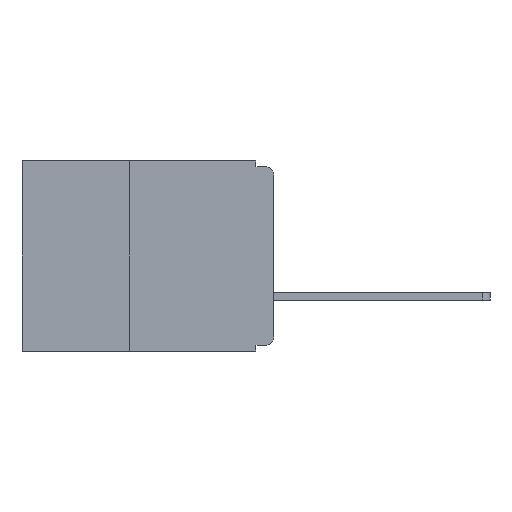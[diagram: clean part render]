
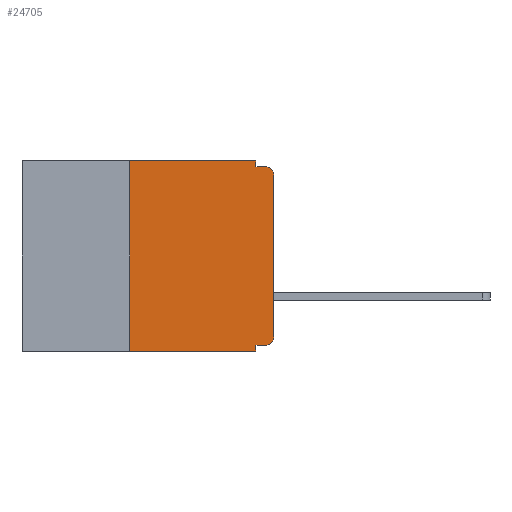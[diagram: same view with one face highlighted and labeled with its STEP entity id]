
A CAD part, left-side view. The second image highlights one B-rep face of the part: STEP entity #24705.
In plain terms, the highlighted planar face has unit normal (-1, 0, 0).
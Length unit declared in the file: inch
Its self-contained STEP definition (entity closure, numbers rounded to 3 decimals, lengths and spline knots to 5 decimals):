
#12 = CARTESIAN_POINT ( 'NONE',  ( 0., 0.031, -0.01 ) ) ;
#156 = VERTEX_POINT ( 'NONE', #18353 ) ;
#365 = EDGE_CURVE ( 'NONE', #24857, #156, #10407, .T. ) ;
#475 = ORIENTED_EDGE ( 'NONE', *, *, #11250, .T. ) ;
#1163 = VERTEX_POINT ( 'NONE', #9125 ) ;
#1238 = AXIS2_PLACEMENT_3D ( 'NONE', #21789, #4111, #19715 ) ;
#1511 = CARTESIAN_POINT ( 'NONE',  ( 0., 0., -0.01 ) ) ;
#2119 = DIRECTION ( 'NONE',  ( 0., 0., 1. ) ) ;
#2271 = FACE_OUTER_BOUND ( 'NONE', #23201, .T. ) ;
#2427 = EDGE_CURVE ( 'NONE', #20034, #23297, #3853, .T. ) ;
#2772 = CIRCLE ( 'NONE', #10408, 0.015 ) ;
#2891 = VERTEX_POINT ( 'NONE', #18834 ) ;
#3417 = CARTESIAN_POINT ( 'NONE',  ( 0., 0.437, 0. ) ) ;
#3722 = ORIENTED_EDGE ( 'NONE', *, *, #5728, .T. ) ;
#3853 = LINE ( 'NONE', #24608, #10629 ) ;
#4111 = DIRECTION ( 'NONE',  ( 1., 0., 0. ) ) ;
#4573 = LINE ( 'NONE', #6805, #6740 ) ;
#4807 = CARTESIAN_POINT ( 'NONE',  ( 0., 0.015, -0.305 ) ) ;
#5728 = EDGE_CURVE ( 'NONE', #15948, #16632, #4573, .T. ) ;
#5747 = VECTOR ( 'NONE', #25563, 39.37008 ) ;
#6016 = ORIENTED_EDGE ( 'NONE', *, *, #365, .F. ) ;
#6680 = CARTESIAN_POINT ( 'NONE',  ( 0., 0.25, -0.33 ) ) ;
#6740 = VECTOR ( 'NONE', #2119, 39.37008 ) ;
#6805 = CARTESIAN_POINT ( 'NONE',  ( 0., 0., 0. ) ) ;
#7125 = CARTESIAN_POINT ( 'NONE',  ( 0., 0., -0.025 ) ) ;
#7126 = DIRECTION ( 'NONE',  ( 0., 0., -1. ) ) ;
#7521 = DIRECTION ( 'NONE',  ( -1., 0., 0. ) ) ;
#8310 = LINE ( 'NONE', #8464, #13542 ) ;
#8464 = CARTESIAN_POINT ( 'NONE',  ( 0., 0.437, -0.33 ) ) ;
#9125 = CARTESIAN_POINT ( 'NONE',  ( 0., 0.031, -0.33 ) ) ;
#9532 = EDGE_CURVE ( 'NONE', #2891, #18909, #24027, .T. ) ;
#10407 = LINE ( 'NONE', #26718, #21393 ) ;
#10408 = AXIS2_PLACEMENT_3D ( 'NONE', #4807, #20368, #7126 ) ;
#10629 = VECTOR ( 'NONE', #24596, 39.37008 ) ;
#11250 = EDGE_CURVE ( 'NONE', #24857, #15948, #2772, .T. ) ;
#11747 = LINE ( 'NONE', #3417, #5747 ) ;
#12354 = ORIENTED_EDGE ( 'NONE', *, *, #22501, .F. ) ;
#12846 = LINE ( 'NONE', #1511, #18021 ) ;
#12863 = DIRECTION ( 'NONE',  ( 0., -1., 0. ) ) ;
#12937 = DIRECTION ( 'NONE',  ( 0., -1., 0. ) ) ;
#13099 = PLANE ( 'NONE',  #1238 ) ;
#13159 = CARTESIAN_POINT ( 'NONE',  ( 0., 0.25, 0. ) ) ;
#13542 = VECTOR ( 'NONE', #12937, 39.37008 ) ;
#13826 = DIRECTION ( 'NONE',  ( 0., 1., 0. ) ) ;
#14186 = VECTOR ( 'NONE', #26689, 39.37008 ) ;
#14560 = ORIENTED_EDGE ( 'NONE', *, *, #27344, .F. ) ;
#14620 = CIRCLE ( 'NONE', #27877, 0.015 ) ;
#14869 = ORIENTED_EDGE ( 'NONE', *, *, #15705, .T. ) ;
#15680 = ORIENTED_EDGE ( 'NONE', *, *, #2427, .F. ) ;
#15705 = EDGE_CURVE ( 'NONE', #20034, #1163, #8310, .T. ) ;
#15948 = VERTEX_POINT ( 'NONE', #22367 ) ;
#16632 = VERTEX_POINT ( 'NONE', #7125 ) ;
#18021 = VECTOR ( 'NONE', #12863, 39.37008 ) ;
#18306 = VECTOR ( 'NONE', #19041, 39.37008 ) ;
#18353 = CARTESIAN_POINT ( 'NONE',  ( 0., 0.031, -0.32 ) ) ;
#18834 = CARTESIAN_POINT ( 'NONE',  ( 0., 0.031, 0. ) ) ;
#18909 = VERTEX_POINT ( 'NONE', #12 ) ;
#19041 = DIRECTION ( 'NONE',  ( 0., 0., -1. ) ) ;
#19715 = DIRECTION ( 'NONE',  ( 0., 0., -1. ) ) ;
#20034 = VERTEX_POINT ( 'NONE', #6680 ) ;
#20327 = ORIENTED_EDGE ( 'NONE', *, *, #21478, .F. ) ;
#20368 = DIRECTION ( 'NONE',  ( -1., 0., 0. ) ) ;
#20774 = CARTESIAN_POINT ( 'NONE',  ( 0., 0.015, -0.025 ) ) ;
#20778 = EDGE_CURVE ( 'NONE', #16632, #27079, #14620, .T. ) ;
#21233 = CARTESIAN_POINT ( 'NONE',  ( 0., 0.031, 0. ) ) ;
#21393 = VECTOR ( 'NONE', #13826, 39.37008 ) ;
#21478 = EDGE_CURVE ( 'NONE', #18909, #27079, #12846, .T. ) ;
#21789 = CARTESIAN_POINT ( 'NONE',  ( 0., 0.437, 0. ) ) ;
#22035 = LINE ( 'NONE', #24540, #14186 ) ;
#22254 = CARTESIAN_POINT ( 'NONE',  ( 0., 0.015, -0.32 ) ) ;
#22367 = CARTESIAN_POINT ( 'NONE',  ( 0., 0., -0.305 ) ) ;
#22501 = EDGE_CURVE ( 'NONE', #23297, #2891, #11747, .T. ) ;
#22907 = DIRECTION ( 'NONE',  ( 0., 0., -1. ) ) ;
#23201 = EDGE_LOOP ( 'NONE', ( #3722, #28403, #20327, #23568, #12354, #15680, #14869, #14560, #6016, #475 ) ) ;
#23297 = VERTEX_POINT ( 'NONE', #13159 ) ;
#23568 = ORIENTED_EDGE ( 'NONE', *, *, #9532, .F. ) ;
#24027 = LINE ( 'NONE', #21233, #18306 ) ;
#24540 = CARTESIAN_POINT ( 'NONE',  ( 0., 0.031, -0.33 ) ) ;
#24596 = DIRECTION ( 'NONE',  ( 0., 0., 1. ) ) ;
#24608 = CARTESIAN_POINT ( 'NONE',  ( 0., 0.25, -0.33 ) ) ;
#24705 = ADVANCED_FACE ( 'NONE', ( #2271 ), #13099, .F. ) ;
#24857 = VERTEX_POINT ( 'NONE', #22254 ) ;
#25563 = DIRECTION ( 'NONE',  ( 0., -1., 0. ) ) ;
#25775 = CARTESIAN_POINT ( 'NONE',  ( 0., 0.015, -0.01 ) ) ;
#26689 = DIRECTION ( 'NONE',  ( 0., 0., -1. ) ) ;
#26718 = CARTESIAN_POINT ( 'NONE',  ( 0., 0., -0.32 ) ) ;
#27079 = VERTEX_POINT ( 'NONE', #25775 ) ;
#27344 = EDGE_CURVE ( 'NONE', #156, #1163, #22035, .T. ) ;
#27877 = AXIS2_PLACEMENT_3D ( 'NONE', #20774, #7521, #22907 ) ;
#28403 = ORIENTED_EDGE ( 'NONE', *, *, #20778, .T. ) ;
